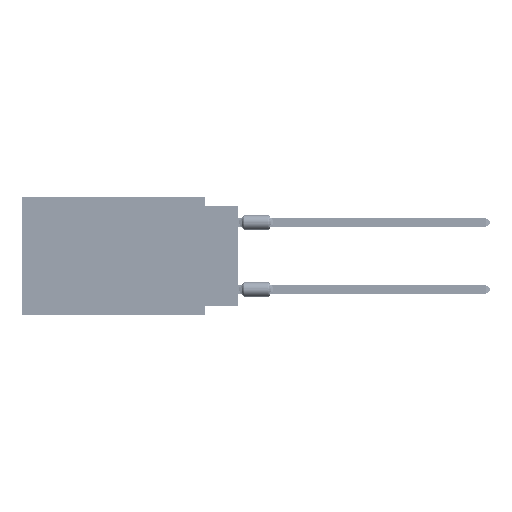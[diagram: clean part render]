
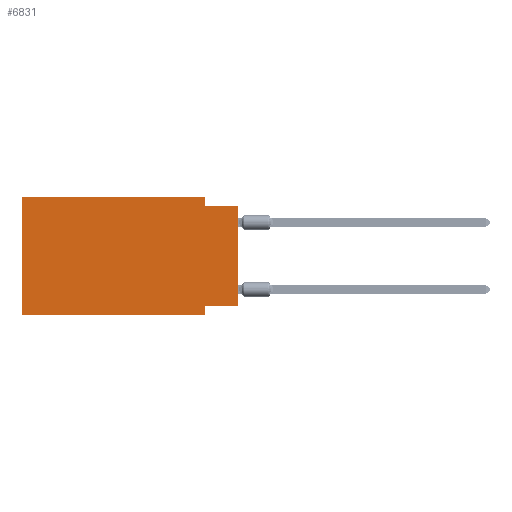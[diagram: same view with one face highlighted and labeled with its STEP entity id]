
A CAD part, left-side view. The second image highlights one B-rep face of the part: STEP entity #6831.
In plain terms, the highlighted planar face has unit normal (-1, 0, 0).
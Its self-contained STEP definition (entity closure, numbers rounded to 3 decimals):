
#628 = LINE ( 'NONE', #61712, #64742 ) ;
#1326 = VERTEX_POINT ( 'NONE', #58858 ) ;
#3911 = LINE ( 'NONE', #41753, #24146 ) ;
#4151 = LINE ( 'NONE', #5393, #28536 ) ;
#4981 = DIRECTION ( 'NONE',  ( 0., 0., 1. ) ) ;
#5393 = CARTESIAN_POINT ( 'NONE',  ( 0., 16.383, 0. ) ) ;
#6332 = VERTEX_POINT ( 'NONE', #43370 ) ;
#6831 = ADVANCED_FACE ( 'NONE', ( #23510 ), #36974, .F. ) ;
#7101 = CARTESIAN_POINT ( 'NONE',  ( 0., 0., -8.255 ) ) ;
#7473 = VERTEX_POINT ( 'NONE', #46797 ) ;
#7930 = CARTESIAN_POINT ( 'NONE',  ( 0., 16.383, -8.89 ) ) ;
#9182 = LINE ( 'NONE', #7930, #56168 ) ;
#9398 = DIRECTION ( 'NONE',  ( 0., 0., -1. ) ) ;
#11545 = CARTESIAN_POINT ( 'NONE',  ( 0., 2.54, -8.89 ) ) ;
#13499 = CARTESIAN_POINT ( 'NONE',  ( 0., 2.54, 0. ) ) ;
#16599 = ORIENTED_EDGE ( 'NONE', *, *, #63374, .F. ) ;
#19256 = ORIENTED_EDGE ( 'NONE', *, *, #57496, .F. ) ;
#20540 = DIRECTION ( 'NONE',  ( 0., 1., 0. ) ) ;
#20822 = ORIENTED_EDGE ( 'NONE', *, *, #24721, .T. ) ;
#20988 = CARTESIAN_POINT ( 'NONE',  ( 0., 16.383, 0. ) ) ;
#22630 = VERTEX_POINT ( 'NONE', #32546 ) ;
#22734 = EDGE_CURVE ( 'NONE', #24364, #36467, #3911, .T. ) ;
#23510 = FACE_OUTER_BOUND ( 'NONE', #72606, .T. ) ;
#24146 = VECTOR ( 'NONE', #9398, 1000. ) ;
#24364 = VERTEX_POINT ( 'NONE', #67748 ) ;
#24542 = VECTOR ( 'NONE', #20540, 1000. ) ;
#24721 = EDGE_CURVE ( 'NONE', #22630, #36467, #9182, .T. ) ;
#27303 = AXIS2_PLACEMENT_3D ( 'NONE', #74378, #36557, #35327 ) ;
#28492 = DIRECTION ( 'NONE',  ( 0., -1., 0. ) ) ;
#28536 = VECTOR ( 'NONE', #50366, 1000. ) ;
#29844 = CARTESIAN_POINT ( 'NONE',  ( 0., 16.383, 0. ) ) ;
#31789 = CARTESIAN_POINT ( 'NONE',  ( 0., 0., -0.635 ) ) ;
#32546 = CARTESIAN_POINT ( 'NONE',  ( 0., 16.383, -8.89 ) ) ;
#32836 = LINE ( 'NONE', #13499, #41316 ) ;
#34719 = ORIENTED_EDGE ( 'NONE', *, *, #70699, .F. ) ;
#35327 = DIRECTION ( 'NONE',  ( 0., 0., -1. ) ) ;
#36467 = VERTEX_POINT ( 'NONE', #11545 ) ;
#36557 = DIRECTION ( 'NONE',  ( 1., 0., 0. ) ) ;
#36974 = PLANE ( 'NONE',  #27303 ) ;
#41316 = VECTOR ( 'NONE', #58465, 1000. ) ;
#41753 = CARTESIAN_POINT ( 'NONE',  ( 0., 2.54, -8.89 ) ) ;
#42873 = LINE ( 'NONE', #29844, #69883 ) ;
#43370 = CARTESIAN_POINT ( 'NONE',  ( 0., 0., -0.635 ) ) ;
#46797 = CARTESIAN_POINT ( 'NONE',  ( 0., 2.54, 0. ) ) ;
#50366 = DIRECTION ( 'NONE',  ( 0., -1., 0. ) ) ;
#50741 = ORIENTED_EDGE ( 'NONE', *, *, #78568, .F. ) ;
#56168 = VECTOR ( 'NONE', #28492, 1000. ) ;
#57496 = EDGE_CURVE ( 'NONE', #7473, #74199, #32836, .T. ) ;
#57700 = VECTOR ( 'NONE', #83065, 1000. ) ;
#58117 = ORIENTED_EDGE ( 'NONE', *, *, #74403, .F. ) ;
#58465 = DIRECTION ( 'NONE',  ( 0., 0., -1. ) ) ;
#58858 = CARTESIAN_POINT ( 'NONE',  ( 0., 0., -8.255 ) ) ;
#61712 = CARTESIAN_POINT ( 'NONE',  ( 0., 0., 0. ) ) ;
#61920 = ORIENTED_EDGE ( 'NONE', *, *, #22734, .F. ) ;
#63349 = EDGE_CURVE ( 'NONE', #1326, #6332, #628, .T. ) ;
#63374 = EDGE_CURVE ( 'NONE', #66324, #7473, #4151, .T. ) ;
#63405 = CARTESIAN_POINT ( 'NONE',  ( 0., 2.54, -0.635 ) ) ;
#64742 = VECTOR ( 'NONE', #4981, 1000. ) ;
#65903 = LINE ( 'NONE', #7101, #24542 ) ;
#66324 = VERTEX_POINT ( 'NONE', #20988 ) ;
#67748 = CARTESIAN_POINT ( 'NONE',  ( 0., 2.54, -8.255 ) ) ;
#68477 = DIRECTION ( 'NONE',  ( 0., 0., 1. ) ) ;
#69320 = ORIENTED_EDGE ( 'NONE', *, *, #63349, .T. ) ;
#69883 = VECTOR ( 'NONE', #68477, 1000. ) ;
#70009 = LINE ( 'NONE', #31789, #57700 ) ;
#70699 = EDGE_CURVE ( 'NONE', #22630, #66324, #42873, .T. ) ;
#72606 = EDGE_LOOP ( 'NONE', ( #69320, #50741, #19256, #16599, #34719, #20822, #61920, #58117 ) ) ;
#74199 = VERTEX_POINT ( 'NONE', #63405 ) ;
#74378 = CARTESIAN_POINT ( 'NONE',  ( 0., 16.383, 0. ) ) ;
#74403 = EDGE_CURVE ( 'NONE', #1326, #24364, #65903, .T. ) ;
#78568 = EDGE_CURVE ( 'NONE', #74199, #6332, #70009, .T. ) ;
#83065 = DIRECTION ( 'NONE',  ( 0., -1., 0. ) ) ;
